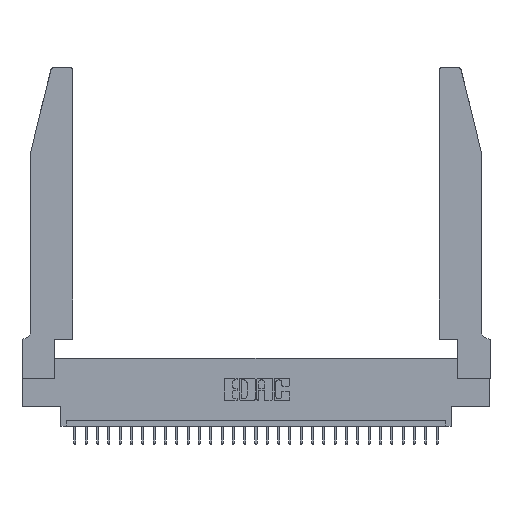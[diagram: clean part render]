
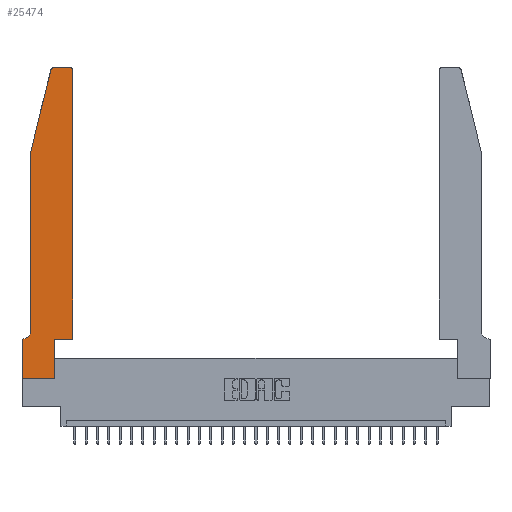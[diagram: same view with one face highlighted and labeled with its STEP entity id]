
A CAD part, top view. The second image highlights one B-rep face of the part: STEP entity #25474.
In plain terms, the highlighted planar face has unit normal (0, 0, 1).
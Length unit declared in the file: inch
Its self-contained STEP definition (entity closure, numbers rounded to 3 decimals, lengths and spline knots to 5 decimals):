
#115 = EDGE_CURVE ( 'NONE', #12276, #25204, #13437, .T. ) ;
#242 = EDGE_CURVE ( 'NONE', #18385, #26120, #7424, .T. ) ;
#457 = VERTEX_POINT ( 'NONE', #23541 ) ;
#721 = DIRECTION ( 'NONE',  ( 1., 0., 0. ) ) ;
#884 = CARTESIAN_POINT ( 'NONE',  ( 0.2865, 0.35, 0.37 ) ) ;
#1123 = DIRECTION ( 'NONE',  ( 1., 0., 0. ) ) ;
#1647 = EDGE_CURVE ( 'NONE', #24466, #9309, #13705, .T. ) ;
#2144 = ORIENTED_EDGE ( 'NONE', *, *, #15428, .T. ) ;
#2639 = EDGE_CURVE ( 'NONE', #26120, #14102, #17023, .T. ) ;
#2770 = ORIENTED_EDGE ( 'NONE', *, *, #21687, .T. ) ;
#2858 = CIRCLE ( 'NONE', #22160, 0.07 ) ;
#2881 = CARTESIAN_POINT ( 'NONE',  ( 0.0755, 2., 0.37 ) ) ;
#3101 = ORIENTED_EDGE ( 'NONE', *, *, #115, .T. ) ;
#3294 = AXIS2_PLACEMENT_3D ( 'NONE', #12822, #17537, #10434 ) ;
#3904 = EDGE_CURVE ( 'NONE', #25204, #23215, #16561, .T. ) ;
#4276 = CARTESIAN_POINT ( 'NONE',  ( 0.4505, 0.35, 0.37 ) ) ;
#4623 = ORIENTED_EDGE ( 'NONE', *, *, #3904, .T. ) ;
#4672 = CARTESIAN_POINT ( 'NONE',  ( 0.4505, 0.35, 0.37 ) ) ;
#4676 = CARTESIAN_POINT ( 'NONE',  ( 0.2865, 0., 0.37 ) ) ;
#4803 = ORIENTED_EDGE ( 'NONE', *, *, #1647, .T. ) ;
#4993 = ORIENTED_EDGE ( 'NONE', *, *, #21123, .T. ) ;
#5333 = VECTOR ( 'NONE', #19159, 39.37008 ) ;
#5729 = CARTESIAN_POINT ( 'NONE',  ( 0.0055, 0.35, 0.37 ) ) ;
#6660 = CARTESIAN_POINT ( 'NONE',  ( 0., 0.35, 0.37 ) ) ;
#7158 = VECTOR ( 'NONE', #18772, 39.37008 ) ;
#7424 = LINE ( 'NONE', #10851, #22392 ) ;
#7566 = DIRECTION ( 'NONE',  ( 0., 0., -1. ) ) ;
#8614 = DIRECTION ( 'NONE',  ( 0., 1., 0. ) ) ;
#9309 = VERTEX_POINT ( 'NONE', #4672 ) ;
#9321 = CARTESIAN_POINT ( 'NONE',  ( 0.4505, 2.72, 0.37 ) ) ;
#9380 = CARTESIAN_POINT ( 'NONE',  ( 0.284, 2.75, 0.37 ) ) ;
#9433 = ORIENTED_EDGE ( 'NONE', *, *, #242, .T. ) ;
#9748 = EDGE_CURVE ( 'NONE', #14102, #24466, #18392, .T. ) ;
#10062 = VERTEX_POINT ( 'NONE', #12307 ) ;
#10434 = DIRECTION ( 'NONE',  ( 1., 0., 0. ) ) ;
#10851 = CARTESIAN_POINT ( 'NONE',  ( 0., 0., 0.37 ) ) ;
#10857 = CARTESIAN_POINT ( 'NONE',  ( 0.0755, 0.35, 0.37 ) ) ;
#10858 = EDGE_LOOP ( 'NONE', ( #4623, #2144, #4993, #2770, #18317, #12131, #9433, #27031, #28515, #4803, #27862, #3101 ) ) ;
#11302 = VECTOR ( 'NONE', #15359, 39.37008 ) ;
#11462 = VECTOR ( 'NONE', #20963, 39.37008 ) ;
#11672 = LINE ( 'NONE', #25735, #7158 ) ;
#11695 = VECTOR ( 'NONE', #15966, 39.37008 ) ;
#12131 = ORIENTED_EDGE ( 'NONE', *, *, #21722, .T. ) ;
#12218 = DIRECTION ( 'NONE',  ( 1., 0., 0. ) ) ;
#12276 = VERTEX_POINT ( 'NONE', #9321 ) ;
#12307 = CARTESIAN_POINT ( 'NONE',  ( 0.0755, 0.42, 0.37 ) ) ;
#12822 = CARTESIAN_POINT ( 'NONE',  ( 0.4205, 2.72, 0.37 ) ) ;
#13270 = PLANE ( 'NONE',  #25836 ) ;
#13437 = CIRCLE ( 'NONE', #3294, 0.03 ) ;
#13705 = LINE ( 'NONE', #4276, #11462 ) ;
#14045 = CARTESIAN_POINT ( 'NONE',  ( 0.0055, 0.42, 0.37 ) ) ;
#14102 = VERTEX_POINT ( 'NONE', #4676 ) ;
#14245 = DIRECTION ( 'NONE',  ( -1., 0., 0. ) ) ;
#15359 = DIRECTION ( 'NONE',  ( -1., 0., 0. ) ) ;
#15428 = EDGE_CURVE ( 'NONE', #23215, #457, #21756, .T. ) ;
#15577 = CARTESIAN_POINT ( 'NONE',  ( 0.0755, 2., 0.37 ) ) ;
#15966 = DIRECTION ( 'NONE',  ( -0.239, -0.971, 0. ) ) ;
#16561 = LINE ( 'NONE', #21629, #5333 ) ;
#17023 = LINE ( 'NONE', #26945, #21839 ) ;
#17537 = DIRECTION ( 'NONE',  ( 0., 0., 1. ) ) ;
#18317 = ORIENTED_EDGE ( 'NONE', *, *, #19077, .T. ) ;
#18385 = VERTEX_POINT ( 'NONE', #6660 ) ;
#18392 = LINE ( 'NONE', #22898, #21355 ) ;
#18414 = LINE ( 'NONE', #15577, #28477 ) ;
#18772 = DIRECTION ( 'NONE',  ( 0., 1., 0. ) ) ;
#19077 = EDGE_CURVE ( 'NONE', #10062, #19786, #2858, .T. ) ;
#19159 = DIRECTION ( 'NONE',  ( -1., 0., 0. ) ) ;
#19786 = VERTEX_POINT ( 'NONE', #5729 ) ;
#19897 = LINE ( 'NONE', #10857, #11302 ) ;
#20327 = CARTESIAN_POINT ( 'NONE',  ( 0., 0., 0.37 ) ) ;
#20431 = DIRECTION ( 'NONE',  ( 0., -1., 0. ) ) ;
#20557 = DIRECTION ( 'NONE',  ( 0., 0., 1. ) ) ;
#20625 = LINE ( 'NONE', #30239, #11695 ) ;
#20963 = DIRECTION ( 'NONE',  ( 1., 0., 0. ) ) ;
#21123 = EDGE_CURVE ( 'NONE', #457, #26403, #20625, .T. ) ;
#21355 = VECTOR ( 'NONE', #8614, 39.37008 ) ;
#21629 = CARTESIAN_POINT ( 'NONE',  ( 0.2605, 2.75, 0.37 ) ) ;
#21687 = EDGE_CURVE ( 'NONE', #26403, #10062, #18414, .T. ) ;
#21699 = DIRECTION ( 'NONE',  ( 0., 0., 1. ) ) ;
#21722 = EDGE_CURVE ( 'NONE', #19786, #18385, #19897, .T. ) ;
#21756 = CIRCLE ( 'NONE', #26055, 0.03 ) ;
#21839 = VECTOR ( 'NONE', #721, 39.37008 ) ;
#22027 = EDGE_CURVE ( 'NONE', #9309, #12276, #11672, .T. ) ;
#22160 = AXIS2_PLACEMENT_3D ( 'NONE', #14045, #7566, #14245 ) ;
#22392 = VECTOR ( 'NONE', #20431, 39.37008 ) ;
#22793 = FACE_OUTER_BOUND ( 'NONE', #10858, .T. ) ;
#22844 = CARTESIAN_POINT ( 'NONE',  ( 0., 0.35, 0.37 ) ) ;
#22898 = CARTESIAN_POINT ( 'NONE',  ( 0.2865, 0.35, 0.37 ) ) ;
#23215 = VERTEX_POINT ( 'NONE', #9380 ) ;
#23541 = CARTESIAN_POINT ( 'NONE',  ( 0.25487, 2.72718, 0.37 ) ) ;
#24466 = VERTEX_POINT ( 'NONE', #884 ) ;
#25204 = VERTEX_POINT ( 'NONE', #30191 ) ;
#25474 = ADVANCED_FACE ( 'NONE', ( #22793 ), #13270, .T. ) ;
#25735 = CARTESIAN_POINT ( 'NONE',  ( 0.4505, 0.35, 0.37 ) ) ;
#25836 = AXIS2_PLACEMENT_3D ( 'NONE', #22844, #20557, #1123 ) ;
#26055 = AXIS2_PLACEMENT_3D ( 'NONE', #26194, #21699, #12218 ) ;
#26120 = VERTEX_POINT ( 'NONE', #20327 ) ;
#26194 = CARTESIAN_POINT ( 'NONE',  ( 0.284, 2.72, 0.37 ) ) ;
#26403 = VERTEX_POINT ( 'NONE', #2881 ) ;
#26945 = CARTESIAN_POINT ( 'NONE',  ( 0., 0., 0.37 ) ) ;
#27031 = ORIENTED_EDGE ( 'NONE', *, *, #2639, .T. ) ;
#27221 = DIRECTION ( 'NONE',  ( 0., -1., 0. ) ) ;
#27862 = ORIENTED_EDGE ( 'NONE', *, *, #22027, .T. ) ;
#28477 = VECTOR ( 'NONE', #27221, 39.37008 ) ;
#28515 = ORIENTED_EDGE ( 'NONE', *, *, #9748, .T. ) ;
#30191 = CARTESIAN_POINT ( 'NONE',  ( 0.4205, 2.75, 0.37 ) ) ;
#30239 = CARTESIAN_POINT ( 'NONE',  ( 0.0755, 2., 0.37 ) ) ;
